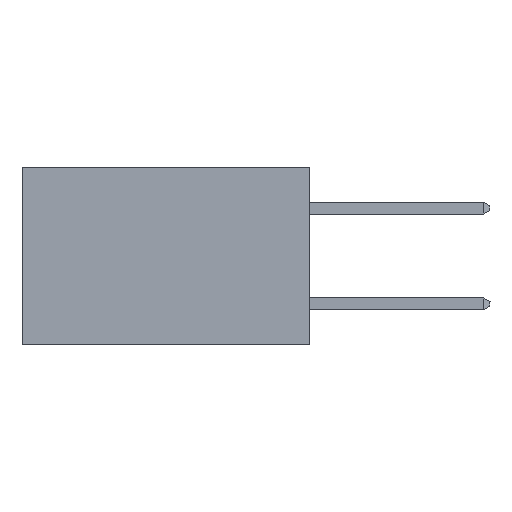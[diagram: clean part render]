
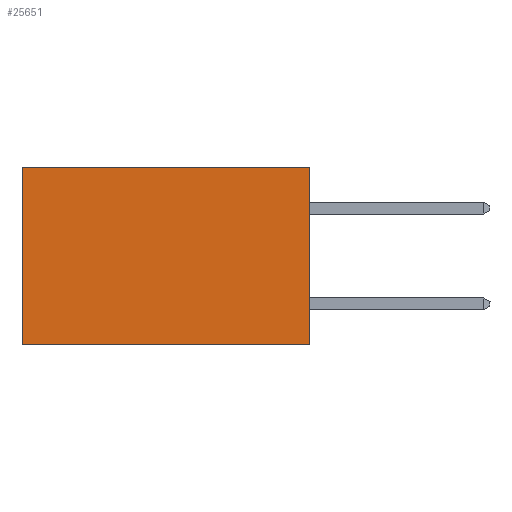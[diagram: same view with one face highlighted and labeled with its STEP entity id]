
A CAD part, left-side view. The second image highlights one B-rep face of the part: STEP entity #25651.
In plain terms, the highlighted planar face has unit normal (-1, 0, 0).
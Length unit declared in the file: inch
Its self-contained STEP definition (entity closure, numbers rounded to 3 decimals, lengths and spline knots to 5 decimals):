
#102 = AXIS2_PLACEMENT_3D ( 'NONE', #35177, #22783, #10662 ) ;
#490 = VERTEX_POINT ( 'NONE', #9337 ) ;
#528 = EDGE_CURVE ( 'NONE', #18592, #38634, #23673, .T. ) ;
#1236 = EDGE_CURVE ( 'NONE', #38634, #37318, #23152, .T. ) ;
#2106 = EDGE_CURVE ( 'NONE', #490, #37318, #33919, .T. ) ;
#2145 = CARTESIAN_POINT ( 'NONE',  ( 0.2875, 0., -0.37 ) ) ;
#2666 = VECTOR ( 'NONE', #18667, 39.37008 ) ;
#4487 = ORIENTED_EDGE ( 'NONE', *, *, #2106, .F. ) ;
#6158 = ORIENTED_EDGE ( 'NONE', *, *, #1236, .T. ) ;
#6865 = ORIENTED_EDGE ( 'NONE', *, *, #23447, .F. ) ;
#6944 = VECTOR ( 'NONE', #20820, 39.37008 ) ;
#7976 = CARTESIAN_POINT ( 'NONE',  ( 0.2875, 0., 0. ) ) ;
#9337 = CARTESIAN_POINT ( 'NONE',  ( 0.2875, 0., -0.37 ) ) ;
#10662 = DIRECTION ( 'NONE',  ( 0., 0., -1. ) ) ;
#11994 = CARTESIAN_POINT ( 'NONE',  ( 0.2875, 0.6, -0.37 ) ) ;
#14971 = LINE ( 'NONE', #7976, #6944 ) ;
#17954 = CARTESIAN_POINT ( 'NONE',  ( 0.2875, 0., 0. ) ) ;
#18486 = DIRECTION ( 'NONE',  ( 0., 1., 0. ) ) ;
#18592 = VERTEX_POINT ( 'NONE', #22117 ) ;
#18667 = DIRECTION ( 'NONE',  ( 0., 0., -1. ) ) ;
#20289 = ORIENTED_EDGE ( 'NONE', *, *, #528, .T. ) ;
#20820 = DIRECTION ( 'NONE',  ( 0., 0., -1. ) ) ;
#21775 = EDGE_LOOP ( 'NONE', ( #6158, #4487, #6865, #20289 ) ) ;
#22117 = CARTESIAN_POINT ( 'NONE',  ( 0.2875, 0., 0. ) ) ;
#22716 = VECTOR ( 'NONE', #18486, 39.37008 ) ;
#22783 = DIRECTION ( 'NONE',  ( 1., 0., 0. ) ) ;
#23152 = LINE ( 'NONE', #25090, #2666 ) ;
#23447 = EDGE_CURVE ( 'NONE', #18592, #490, #14971, .T. ) ;
#23557 = CARTESIAN_POINT ( 'NONE',  ( 0.2875, 0.6, 0. ) ) ;
#23673 = LINE ( 'NONE', #17954, #22716 ) ;
#24493 = VECTOR ( 'NONE', #32110, 39.37008 ) ;
#25090 = CARTESIAN_POINT ( 'NONE',  ( 0.2875, 0.6, 0. ) ) ;
#25651 = ADVANCED_FACE ( 'NONE', ( #28817 ), #26222, .F. ) ;
#26222 = PLANE ( 'NONE',  #102 ) ;
#28817 = FACE_OUTER_BOUND ( 'NONE', #21775, .T. ) ;
#32110 = DIRECTION ( 'NONE',  ( 0., 1., 0. ) ) ;
#33919 = LINE ( 'NONE', #2145, #24493 ) ;
#35177 = CARTESIAN_POINT ( 'NONE',  ( 0.2875, 0., 0. ) ) ;
#37318 = VERTEX_POINT ( 'NONE', #11994 ) ;
#38634 = VERTEX_POINT ( 'NONE', #23557 ) ;
